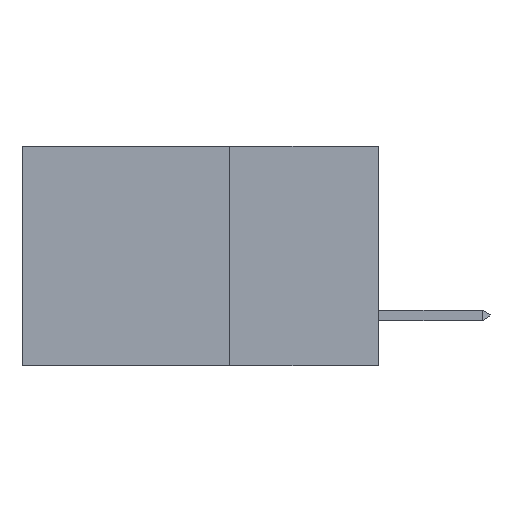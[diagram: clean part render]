
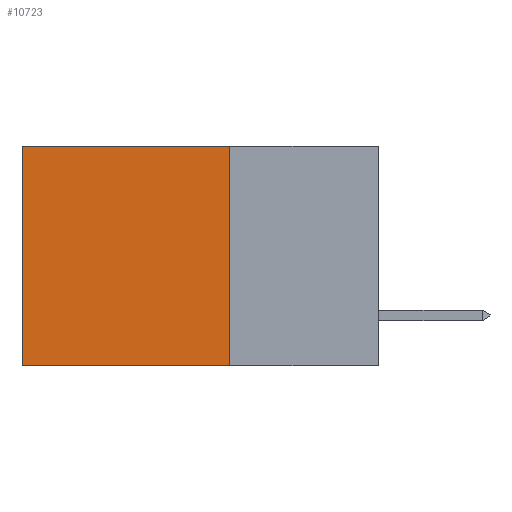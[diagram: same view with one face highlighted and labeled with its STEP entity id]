
A CAD part, left-side view. The second image highlights one B-rep face of the part: STEP entity #10723.
In plain terms, the highlighted planar face has unit normal (-1, 0, 0).
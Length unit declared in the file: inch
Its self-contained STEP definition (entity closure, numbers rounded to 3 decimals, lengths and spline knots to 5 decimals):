
#118 = CARTESIAN_POINT ( 'NONE',  ( 0.2615, 0.25, -0.37 ) ) ;
#458 = DIRECTION ( 'NONE',  ( 0., 1., 0. ) ) ;
#1179 = CARTESIAN_POINT ( 'NONE',  ( 0.2615, 0.6, -0.37 ) ) ;
#2077 = DIRECTION ( 'NONE',  ( 0., 0., -1. ) ) ;
#2590 = ORIENTED_EDGE ( 'NONE', *, *, #16007, .T. ) ;
#3268 = CARTESIAN_POINT ( 'NONE',  ( 0.2615, 0.6, -0.37 ) ) ;
#4035 = LINE ( 'NONE', #18679, #16999 ) ;
#4088 = ORIENTED_EDGE ( 'NONE', *, *, #4720, .T. ) ;
#4649 = PLANE ( 'NONE',  #10192 ) ;
#4720 = EDGE_CURVE ( 'NONE', #13590, #9345, #14010, .T. ) ;
#4741 = CARTESIAN_POINT ( 'NONE',  ( 0.2615, 0.25, -0.37 ) ) ;
#4835 = ORIENTED_EDGE ( 'NONE', *, *, #6817, .F. ) ;
#5570 = DIRECTION ( 'NONE',  ( 0., 1., 0. ) ) ;
#5619 = DIRECTION ( 'NONE',  ( 0., 0., -1. ) ) ;
#6817 = EDGE_CURVE ( 'NONE', #18528, #10700, #9389, .T. ) ;
#7336 = FACE_OUTER_BOUND ( 'NONE', #10190, .T. ) ;
#7613 = DIRECTION ( 'NONE',  ( 0., 0., -1. ) ) ;
#7934 = CARTESIAN_POINT ( 'NONE',  ( 0.2615, 0.25, -0.37 ) ) ;
#9345 = VERTEX_POINT ( 'NONE', #3268 ) ;
#9389 = LINE ( 'NONE', #7934, #13197 ) ;
#10190 = EDGE_LOOP ( 'NONE', ( #4088, #13378, #4835, #2590 ) ) ;
#10192 = AXIS2_PLACEMENT_3D ( 'NONE', #4741, #19025, #7613 ) ;
#10700 = VERTEX_POINT ( 'NONE', #118 ) ;
#10723 = ADVANCED_FACE ( 'NONE', ( #7336 ), #4649, .F. ) ;
#10918 = VECTOR ( 'NONE', #458, 39.37008 ) ;
#12134 = CARTESIAN_POINT ( 'NONE',  ( 0.2615, 0.25, 0. ) ) ;
#12230 = LINE ( 'NONE', #12134, #10918 ) ;
#13082 = EDGE_CURVE ( 'NONE', #10700, #9345, #4035, .T. ) ;
#13197 = VECTOR ( 'NONE', #2077, 39.37008 ) ;
#13378 = ORIENTED_EDGE ( 'NONE', *, *, #13082, .F. ) ;
#13590 = VERTEX_POINT ( 'NONE', #15053 ) ;
#14010 = LINE ( 'NONE', #1179, #15747 ) ;
#15053 = CARTESIAN_POINT ( 'NONE',  ( 0.2615, 0.6, 0. ) ) ;
#15747 = VECTOR ( 'NONE', #5619, 39.37008 ) ;
#16007 = EDGE_CURVE ( 'NONE', #18528, #13590, #12230, .T. ) ;
#16583 = CARTESIAN_POINT ( 'NONE',  ( 0.2615, 0.25, 0. ) ) ;
#16999 = VECTOR ( 'NONE', #5570, 39.37008 ) ;
#18528 = VERTEX_POINT ( 'NONE', #16583 ) ;
#18679 = CARTESIAN_POINT ( 'NONE',  ( 0.2615, 0.25, -0.37 ) ) ;
#19025 = DIRECTION ( 'NONE',  ( 1., 0., 0. ) ) ;
